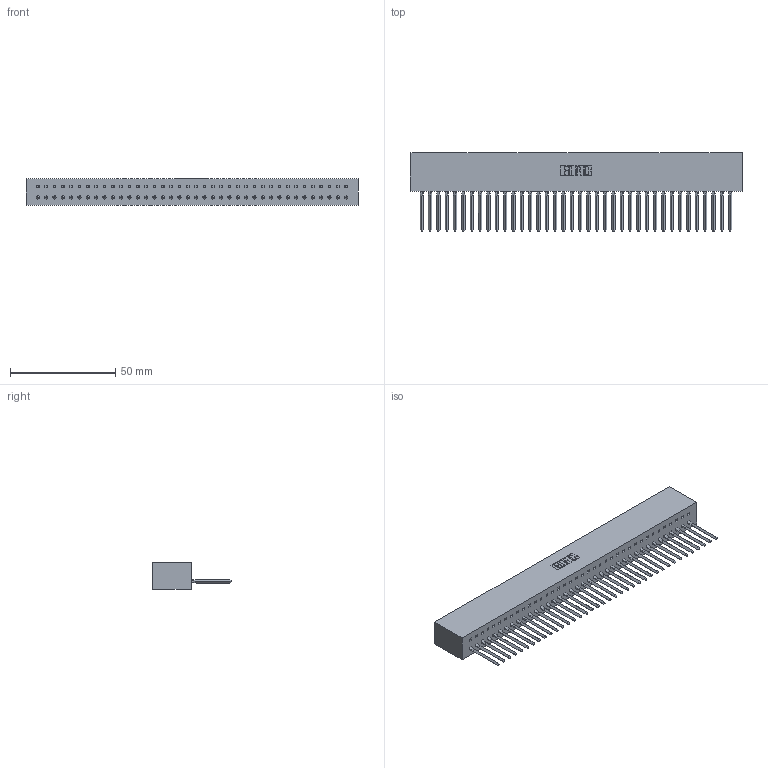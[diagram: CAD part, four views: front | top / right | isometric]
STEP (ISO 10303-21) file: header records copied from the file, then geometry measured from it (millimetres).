
FILE_DESCRIPTION (( 'STEP AP203' ), '1' );
FILE_NAME ('317-038-541-601.STEP', '2020-02-27T23:25:41', ( '' ), ( '' ), 'SwSTEP 2.0', 'SolidWorks 2016', '' );
FILE_SCHEMA (( 'CONFIG_CONTROL_DESIGN' ));
Length unit declared in the file: inch
Products named in the file (3): 317-290-002_541; 317 Part_Lugless; 317-038-541-601
Assembly tree (39 placements, depth 2):
  317-038-541-601
    317 Part_Lugless
    317-290-002_541  x38
Bounding box: 157.78 x 37.34 x 12.7 mm (x, y, z)
Volume: 27170.2 mm3; surface area: 38453.7 mm2
Topology: 39 solids, 39 shells, 5866 faces, 16731 edges, 10874 vertices
Faces by surface type: plane 4762, cylinder 952, bspline 152
Entity records: 55410 total; most frequent: CARTESIAN_POINT 10491, ORIENTED_EDGE 9782, DIRECTION 8023, EDGE_CURVE 4891, VECTOR 4535, LINE 4535, VERTEX_POINT 3252, AXIS2_PLACEMENT_3D 1744
